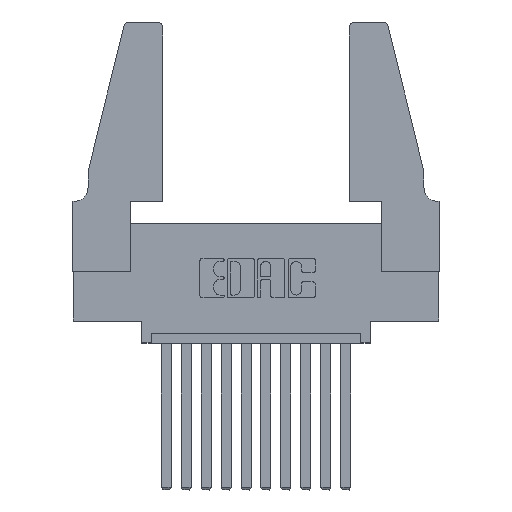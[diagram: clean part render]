
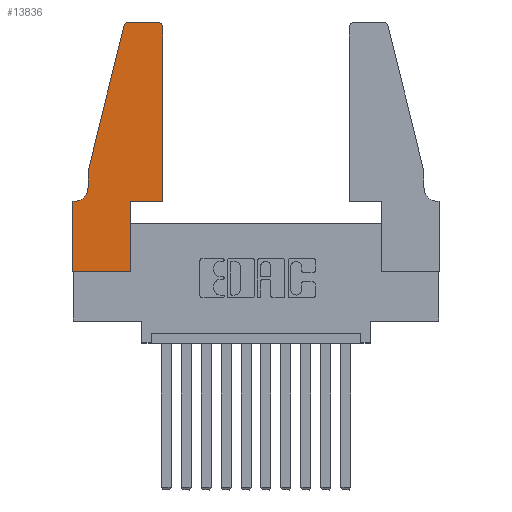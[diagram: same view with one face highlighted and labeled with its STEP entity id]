
A CAD part, top view. The second image highlights one B-rep face of the part: STEP entity #13836.
In plain terms, the highlighted planar face has unit normal (0, 0, 1).
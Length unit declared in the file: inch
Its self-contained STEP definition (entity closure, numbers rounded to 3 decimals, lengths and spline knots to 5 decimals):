
#11 = LINE ( 'NONE', #11903, #9483 ) ;
#245 = EDGE_CURVE ( 'NONE', #2768, #4975, #673, .T. ) ;
#272 = ORIENTED_EDGE ( 'NONE', *, *, #1373, .T. ) ;
#286 = FACE_OUTER_BOUND ( 'NONE', #5606, .T. ) ;
#469 = LINE ( 'NONE', #1316, #4066 ) ;
#503 = DIRECTION ( 'NONE',  ( 0., -1., 0. ) ) ;
#561 = CARTESIAN_POINT ( 'NONE',  ( 0.0755, 0.5, 0.37 ) ) ;
#566 = CARTESIAN_POINT ( 'NONE',  ( 0.25487, 1.22718, 0.37 ) ) ;
#616 = EDGE_CURVE ( 'NONE', #2737, #1613, #3720, .T. ) ;
#673 = CIRCLE ( 'NONE', #7900, 0.03 ) ;
#1020 = VERTEX_POINT ( 'NONE', #9550 ) ;
#1072 = DIRECTION ( 'NONE',  ( 1., 0., 0. ) ) ;
#1225 = ORIENTED_EDGE ( 'NONE', *, *, #616, .T. ) ;
#1316 = CARTESIAN_POINT ( 'NONE',  ( 0.2605, 1.25, 0.37 ) ) ;
#1372 = LINE ( 'NONE', #6542, #4495 ) ;
#1373 = EDGE_CURVE ( 'NONE', #4975, #13715, #469, .T. ) ;
#1613 = VERTEX_POINT ( 'NONE', #7895 ) ;
#1981 = CARTESIAN_POINT ( 'NONE',  ( 0.284, 1.22, 0.37 ) ) ;
#2566 = AXIS2_PLACEMENT_3D ( 'NONE', #13023, #4488, #6808 ) ;
#2737 = VERTEX_POINT ( 'NONE', #7976 ) ;
#2768 = VERTEX_POINT ( 'NONE', #10110 ) ;
#2802 = CARTESIAN_POINT ( 'NONE',  ( 0.4205, 1.25, 0.37 ) ) ;
#2971 = DIRECTION ( 'NONE',  ( 1., 0., 0. ) ) ;
#3211 = CARTESIAN_POINT ( 'NONE',  ( 0.4505, 0.35, 0.37 ) ) ;
#3263 = ORIENTED_EDGE ( 'NONE', *, *, #4746, .T. ) ;
#3265 = EDGE_CURVE ( 'NONE', #12748, #1020, #6907, .T. ) ;
#3425 = EDGE_CURVE ( 'NONE', #13945, #11201, #13614, .T. ) ;
#3720 = LINE ( 'NONE', #6993, #9093 ) ;
#3977 = LINE ( 'NONE', #3211, #9849 ) ;
#4066 = VECTOR ( 'NONE', #9604, 39.37008 ) ;
#4449 = CARTESIAN_POINT ( 'NONE',  ( 0.0755, 0.5, 0.37 ) ) ;
#4484 = ORIENTED_EDGE ( 'NONE', *, *, #3425, .T. ) ;
#4488 = DIRECTION ( 'NONE',  ( 0., 0., -1. ) ) ;
#4495 = VECTOR ( 'NONE', #8669, 39.37008 ) ;
#4523 = DIRECTION ( 'NONE',  ( 0., 0., 1. ) ) ;
#4601 = DIRECTION ( 'NONE',  ( 0., 0., 1. ) ) ;
#4746 = EDGE_CURVE ( 'NONE', #13954, #5149, #5390, .T. ) ;
#4881 = DIRECTION ( 'NONE',  ( 0., 1., 0. ) ) ;
#4975 = VERTEX_POINT ( 'NONE', #2802 ) ;
#5001 = LINE ( 'NONE', #7525, #12176 ) ;
#5149 = VERTEX_POINT ( 'NONE', #561 ) ;
#5390 = LINE ( 'NONE', #4449, #13221 ) ;
#5606 = EDGE_LOOP ( 'NONE', ( #272, #10734, #3263, #9961, #4484, #13820, #1225, #9791, #13577, #10158, #6277, #13345 ) ) ;
#5617 = LINE ( 'NONE', #11499, #12391 ) ;
#6140 = DIRECTION ( 'NONE',  ( -0.239, -0.971, 0. ) ) ;
#6222 = CARTESIAN_POINT ( 'NONE',  ( 0.284, 1.25, 0.37 ) ) ;
#6277 = ORIENTED_EDGE ( 'NONE', *, *, #7827, .T. ) ;
#6542 = CARTESIAN_POINT ( 'NONE',  ( 0.0755, 0.5, 0.37 ) ) ;
#6623 = EDGE_CURVE ( 'NONE', #13715, #13954, #7840, .T. ) ;
#6700 = CARTESIAN_POINT ( 'NONE',  ( 0.4205, 1.22, 0.37 ) ) ;
#6808 = DIRECTION ( 'NONE',  ( -1., 0., 0. ) ) ;
#6907 = LINE ( 'NONE', #10605, #7589 ) ;
#6993 = CARTESIAN_POINT ( 'NONE',  ( 0., 0., 0.37 ) ) ;
#7525 = CARTESIAN_POINT ( 'NONE',  ( 0., 0., 0.37 ) ) ;
#7589 = VECTOR ( 'NONE', #13843, 39.37008 ) ;
#7827 = EDGE_CURVE ( 'NONE', #9598, #2768, #11, .T. ) ;
#7840 = CIRCLE ( 'NONE', #13050, 0.03 ) ;
#7895 = CARTESIAN_POINT ( 'NONE',  ( 0., 0., 0.37 ) ) ;
#7900 = AXIS2_PLACEMENT_3D ( 'NONE', #6700, #4601, #12959 ) ;
#7976 = CARTESIAN_POINT ( 'NONE',  ( 0., 0.35, 0.37 ) ) ;
#8341 = EDGE_CURVE ( 'NONE', #11201, #2737, #5617, .T. ) ;
#8401 = DIRECTION ( 'NONE',  ( -1., 0., 0. ) ) ;
#8669 = DIRECTION ( 'NONE',  ( 0., -1., 0. ) ) ;
#9093 = VECTOR ( 'NONE', #503, 39.37008 ) ;
#9390 = CARTESIAN_POINT ( 'NONE',  ( 0.0055, 0.35, 0.37 ) ) ;
#9483 = VECTOR ( 'NONE', #4881, 39.37008 ) ;
#9550 = CARTESIAN_POINT ( 'NONE',  ( 0.2865, 0.35, 0.37 ) ) ;
#9576 = AXIS2_PLACEMENT_3D ( 'NONE', #13145, #4523, #13195 ) ;
#9598 = VERTEX_POINT ( 'NONE', #9962 ) ;
#9604 = DIRECTION ( 'NONE',  ( -1., 0., 0. ) ) ;
#9791 = ORIENTED_EDGE ( 'NONE', *, *, #10342, .T. ) ;
#9845 = PLANE ( 'NONE',  #9576 ) ;
#9849 = VECTOR ( 'NONE', #10739, 39.37008 ) ;
#9961 = ORIENTED_EDGE ( 'NONE', *, *, #10509, .T. ) ;
#9962 = CARTESIAN_POINT ( 'NONE',  ( 0.4505, 0.35, 0.37 ) ) ;
#10110 = CARTESIAN_POINT ( 'NONE',  ( 0.4505, 1.22, 0.37 ) ) ;
#10158 = ORIENTED_EDGE ( 'NONE', *, *, #10205, .T. ) ;
#10205 = EDGE_CURVE ( 'NONE', #1020, #9598, #3977, .T. ) ;
#10322 = CARTESIAN_POINT ( 'NONE',  ( 0.0755, 0.42, 0.37 ) ) ;
#10342 = EDGE_CURVE ( 'NONE', #1613, #12748, #5001, .T. ) ;
#10509 = EDGE_CURVE ( 'NONE', #5149, #13945, #1372, .T. ) ;
#10605 = CARTESIAN_POINT ( 'NONE',  ( 0.2865, 0.35, 0.37 ) ) ;
#10734 = ORIENTED_EDGE ( 'NONE', *, *, #6623, .T. ) ;
#10739 = DIRECTION ( 'NONE',  ( 1., 0., 0. ) ) ;
#11201 = VERTEX_POINT ( 'NONE', #9390 ) ;
#11499 = CARTESIAN_POINT ( 'NONE',  ( 0.0755, 0.35, 0.37 ) ) ;
#11681 = DIRECTION ( 'NONE',  ( 0., 0., 1. ) ) ;
#11903 = CARTESIAN_POINT ( 'NONE',  ( 0.4505, 0.35, 0.37 ) ) ;
#12176 = VECTOR ( 'NONE', #1072, 39.37008 ) ;
#12391 = VECTOR ( 'NONE', #8401, 39.37008 ) ;
#12748 = VERTEX_POINT ( 'NONE', #13078 ) ;
#12959 = DIRECTION ( 'NONE',  ( 1., 0., 0. ) ) ;
#13023 = CARTESIAN_POINT ( 'NONE',  ( 0.0055, 0.42, 0.37 ) ) ;
#13050 = AXIS2_PLACEMENT_3D ( 'NONE', #1981, #11681, #2971 ) ;
#13078 = CARTESIAN_POINT ( 'NONE',  ( 0.2865, 0., 0.37 ) ) ;
#13145 = CARTESIAN_POINT ( 'NONE',  ( 0., 0.35, 0.37 ) ) ;
#13195 = DIRECTION ( 'NONE',  ( 1., 0., 0. ) ) ;
#13221 = VECTOR ( 'NONE', #6140, 39.37008 ) ;
#13345 = ORIENTED_EDGE ( 'NONE', *, *, #245, .T. ) ;
#13577 = ORIENTED_EDGE ( 'NONE', *, *, #3265, .T. ) ;
#13614 = CIRCLE ( 'NONE', #2566, 0.07 ) ;
#13715 = VERTEX_POINT ( 'NONE', #6222 ) ;
#13820 = ORIENTED_EDGE ( 'NONE', *, *, #8341, .T. ) ;
#13836 = ADVANCED_FACE ( 'NONE', ( #286 ), #9845, .T. ) ;
#13843 = DIRECTION ( 'NONE',  ( 0., 1., 0. ) ) ;
#13945 = VERTEX_POINT ( 'NONE', #10322 ) ;
#13954 = VERTEX_POINT ( 'NONE', #566 ) ;
